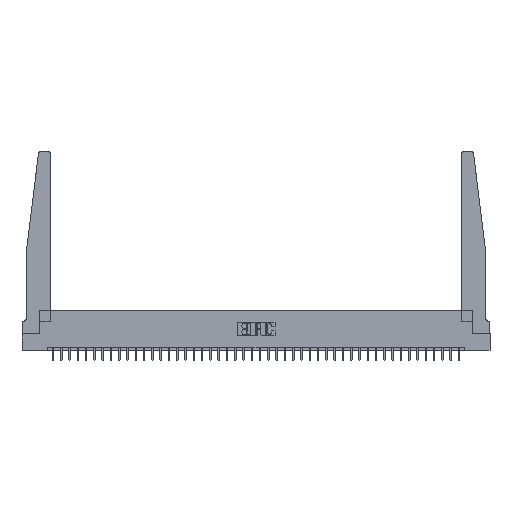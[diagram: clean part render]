
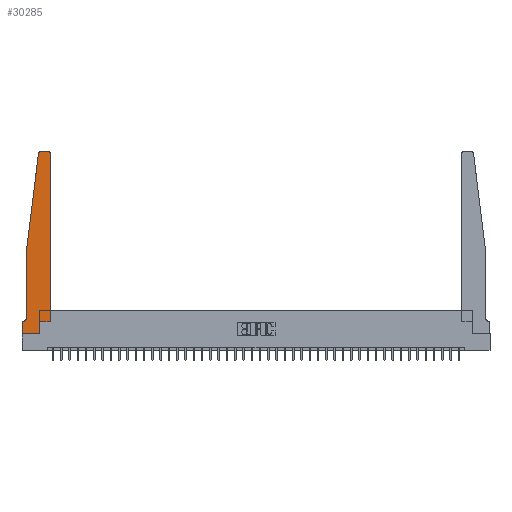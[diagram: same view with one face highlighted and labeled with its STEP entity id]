
A CAD part, top view. The second image highlights one B-rep face of the part: STEP entity #30285.
In plain terms, the highlighted planar face has unit normal (0, 0, 1).
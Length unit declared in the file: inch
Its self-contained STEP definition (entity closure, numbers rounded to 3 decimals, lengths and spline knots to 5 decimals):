
#233 = PLANE ( 'NONE',  #11292 ) ;
#454 = VERTEX_POINT ( 'NONE', #17760 ) ;
#750 = VERTEX_POINT ( 'NONE', #2719 ) ;
#791 = VERTEX_POINT ( 'NONE', #17422 ) ;
#831 = VECTOR ( 'NONE', #21063, 39.37008 ) ;
#967 = DIRECTION ( 'NONE',  ( 1., 0., 0. ) ) ;
#1541 = LINE ( 'NONE', #27269, #1999 ) ;
#1549 = DIRECTION ( 'NONE',  ( 1., 0., 0. ) ) ;
#1747 = DIRECTION ( 'NONE',  ( 1., 0., 0. ) ) ;
#1872 = ORIENTED_EDGE ( 'NONE', *, *, #17129, .T. ) ;
#1999 = VECTOR ( 'NONE', #33042, 39.37008 ) ;
#2046 = CARTESIAN_POINT ( 'NONE',  ( 0.065, 1.25, 0.37 ) ) ;
#2341 = DIRECTION ( 'NONE',  ( 0., 0., 1. ) ) ;
#2677 = DIRECTION ( 'NONE',  ( 0., -1., 0. ) ) ;
#2719 = CARTESIAN_POINT ( 'NONE',  ( 0.015, 0.1875, 0.37 ) ) ;
#2820 = FACE_OUTER_BOUND ( 'NONE', #3216, .T. ) ;
#2966 = EDGE_CURVE ( 'NONE', #750, #21786, #28495, .T. ) ;
#3216 = EDGE_LOOP ( 'NONE', ( #13675, #22680, #20046, #4343, #30601, #10419, #14352, #1872, #5628, #17845, #4630, #26867 ) ) ;
#3575 = EDGE_CURVE ( 'NONE', #14418, #454, #19257, .T. ) ;
#3647 = CARTESIAN_POINT ( 'NONE',  ( 0.2605, 0.18, 0.37 ) ) ;
#4147 = EDGE_CURVE ( 'NONE', #9131, #35243, #26633, .T. ) ;
#4343 = ORIENTED_EDGE ( 'NONE', *, *, #22541, .T. ) ;
#4630 = ORIENTED_EDGE ( 'NONE', *, *, #35709, .T. ) ;
#5096 = VECTOR ( 'NONE', #967, 39.37008 ) ;
#5385 = CARTESIAN_POINT ( 'NONE',  ( 0.395, 2.72, 0.37 ) ) ;
#5628 = ORIENTED_EDGE ( 'NONE', *, *, #22743, .T. ) ;
#5812 = EDGE_CURVE ( 'NONE', #33830, #24562, #12918, .T. ) ;
#6288 = LINE ( 'NONE', #14286, #20411 ) ;
#7192 = DIRECTION ( 'NONE',  ( 0., 1., 0. ) ) ;
#7379 = CARTESIAN_POINT ( 'NONE',  ( 0., 0.1875, 0.37 ) ) ;
#8008 = CARTESIAN_POINT ( 'NONE',  ( 0.065, 1.25, 0.37 ) ) ;
#8612 = AXIS2_PLACEMENT_3D ( 'NONE', #27868, #11324, #25278 ) ;
#9131 = VERTEX_POINT ( 'NONE', #32083 ) ;
#10419 = ORIENTED_EDGE ( 'NONE', *, *, #2966, .T. ) ;
#10992 = DIRECTION ( 'NONE',  ( 1., 0., 0. ) ) ;
#11292 = AXIS2_PLACEMENT_3D ( 'NONE', #27770, #31090, #19928 ) ;
#11324 = DIRECTION ( 'NONE',  ( 0., 0., -1. ) ) ;
#11841 = EDGE_CURVE ( 'NONE', #24562, #9131, #35867, .T. ) ;
#12686 = VECTOR ( 'NONE', #1747, 39.37008 ) ;
#12918 = LINE ( 'NONE', #18933, #17747 ) ;
#13297 = CARTESIAN_POINT ( 'NONE',  ( 0.395, 2.75, 0.37 ) ) ;
#13675 = ORIENTED_EDGE ( 'NONE', *, *, #5812, .T. ) ;
#14286 = CARTESIAN_POINT ( 'NONE',  ( 0.065, 1.25, 0.37 ) ) ;
#14352 = ORIENTED_EDGE ( 'NONE', *, *, #24513, .T. ) ;
#14418 = VERTEX_POINT ( 'NONE', #16317 ) ;
#15397 = DIRECTION ( 'NONE',  ( 0., 0., 1. ) ) ;
#15775 = VERTEX_POINT ( 'NONE', #23426 ) ;
#16317 = CARTESIAN_POINT ( 'NONE',  ( 0.2605, 0.18, 0.37 ) ) ;
#17129 = EDGE_CURVE ( 'NONE', #791, #15775, #30214, .T. ) ;
#17422 = CARTESIAN_POINT ( 'NONE',  ( 0., 0., 0.37 ) ) ;
#17747 = VECTOR ( 'NONE', #33637, 39.37008 ) ;
#17760 = CARTESIAN_POINT ( 'NONE',  ( 0.425, 0.18, 0.37 ) ) ;
#17836 = CARTESIAN_POINT ( 'NONE',  ( 0., 0., 0.37 ) ) ;
#17845 = ORIENTED_EDGE ( 'NONE', *, *, #3575, .T. ) ;
#17918 = CARTESIAN_POINT ( 'NONE',  ( 0.065, 0.1875, 0.37 ) ) ;
#18085 = AXIS2_PLACEMENT_3D ( 'NONE', #23681, #15397, #1549 ) ;
#18613 = CARTESIAN_POINT ( 'NONE',  ( 0.425, 0.18, 0.37 ) ) ;
#18933 = CARTESIAN_POINT ( 'NONE',  ( 0.25, 2.75, 0.37 ) ) ;
#18953 = VERTEX_POINT ( 'NONE', #35484 ) ;
#19077 = VECTOR ( 'NONE', #20653, 39.37008 ) ;
#19175 = VECTOR ( 'NONE', #32771, 39.37008 ) ;
#19257 = LINE ( 'NONE', #18613, #12686 ) ;
#19482 = LINE ( 'NONE', #32628, #34807 ) ;
#19928 = DIRECTION ( 'NONE',  ( 1., 0., 0. ) ) ;
#20046 = ORIENTED_EDGE ( 'NONE', *, *, #4147, .T. ) ;
#20411 = VECTOR ( 'NONE', #2677, 39.37008 ) ;
#20653 = DIRECTION ( 'NONE',  ( 0., 1., 0. ) ) ;
#21063 = DIRECTION ( 'NONE',  ( -1., 0., 0. ) ) ;
#21091 = CIRCLE ( 'NONE', #8612, 0.05 ) ;
#21097 = EDGE_CURVE ( 'NONE', #18953, #750, #21091, .T. ) ;
#21786 = VERTEX_POINT ( 'NONE', #7379 ) ;
#22541 = EDGE_CURVE ( 'NONE', #35243, #18953, #6288, .T. ) ;
#22680 = ORIENTED_EDGE ( 'NONE', *, *, #11841, .T. ) ;
#22743 = EDGE_CURVE ( 'NONE', #15775, #14418, #23448, .T. ) ;
#23426 = CARTESIAN_POINT ( 'NONE',  ( 0.2605, 0., 0.37 ) ) ;
#23448 = LINE ( 'NONE', #3647, #19077 ) ;
#23681 = CARTESIAN_POINT ( 'NONE',  ( 0.27653, 2.72, 0.37 ) ) ;
#24152 = VERTEX_POINT ( 'NONE', #30123 ) ;
#24513 = EDGE_CURVE ( 'NONE', #21786, #791, #1541, .T. ) ;
#24562 = VERTEX_POINT ( 'NONE', #35880 ) ;
#25278 = DIRECTION ( 'NONE',  ( -1., 0., 0. ) ) ;
#26094 = CIRCLE ( 'NONE', #36198, 0.03 ) ;
#26633 = LINE ( 'NONE', #8008, #19175 ) ;
#26867 = ORIENTED_EDGE ( 'NONE', *, *, #31602, .T. ) ;
#27269 = CARTESIAN_POINT ( 'NONE',  ( 0., 0., 0.37 ) ) ;
#27770 = CARTESIAN_POINT ( 'NONE',  ( 0., 0.1875, 0.37 ) ) ;
#27868 = CARTESIAN_POINT ( 'NONE',  ( 0.015, 0.2375, 0.37 ) ) ;
#28495 = LINE ( 'NONE', #17918, #831 ) ;
#30123 = CARTESIAN_POINT ( 'NONE',  ( 0.425, 2.72, 0.37 ) ) ;
#30214 = LINE ( 'NONE', #17836, #5096 ) ;
#30285 = ADVANCED_FACE ( 'NONE', ( #2820 ), #233, .T. ) ;
#30601 = ORIENTED_EDGE ( 'NONE', *, *, #21097, .T. ) ;
#31090 = DIRECTION ( 'NONE',  ( 0., 0., 1. ) ) ;
#31602 = EDGE_CURVE ( 'NONE', #24152, #33830, #26094, .T. ) ;
#32083 = CARTESIAN_POINT ( 'NONE',  ( 0.24675, 2.72367, 0.37 ) ) ;
#32628 = CARTESIAN_POINT ( 'NONE',  ( 0.425, 0.18, 0.37 ) ) ;
#32771 = DIRECTION ( 'NONE',  ( -0.122, -0.992, 0. ) ) ;
#33042 = DIRECTION ( 'NONE',  ( 0., -1., 0. ) ) ;
#33637 = DIRECTION ( 'NONE',  ( -1., 0., 0. ) ) ;
#33830 = VERTEX_POINT ( 'NONE', #13297 ) ;
#34807 = VECTOR ( 'NONE', #7192, 39.37008 ) ;
#35243 = VERTEX_POINT ( 'NONE', #2046 ) ;
#35484 = CARTESIAN_POINT ( 'NONE',  ( 0.065, 0.2375, 0.37 ) ) ;
#35709 = EDGE_CURVE ( 'NONE', #454, #24152, #19482, .T. ) ;
#35867 = CIRCLE ( 'NONE', #18085, 0.03 ) ;
#35880 = CARTESIAN_POINT ( 'NONE',  ( 0.27653, 2.75, 0.37 ) ) ;
#36198 = AXIS2_PLACEMENT_3D ( 'NONE', #5385, #2341, #10992 ) ;
